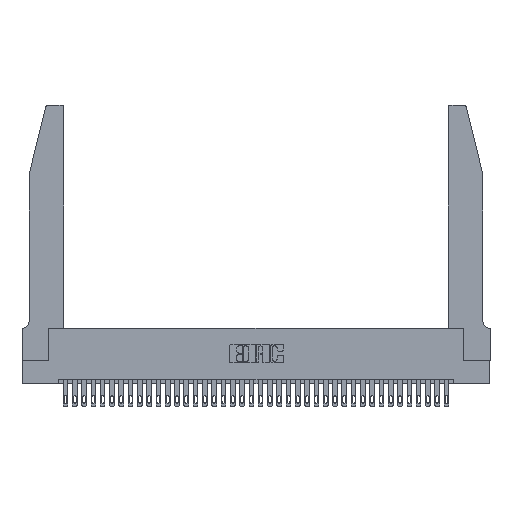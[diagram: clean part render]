
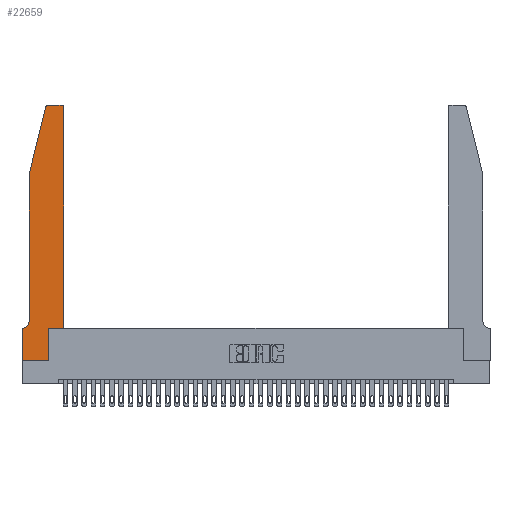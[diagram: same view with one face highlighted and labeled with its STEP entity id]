
A CAD part, top view. The second image highlights one B-rep face of the part: STEP entity #22659.
In plain terms, the highlighted planar face has unit normal (0, 0, 1).
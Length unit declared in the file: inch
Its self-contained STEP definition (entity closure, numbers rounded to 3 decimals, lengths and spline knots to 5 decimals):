
#34 = CARTESIAN_POINT ( 'NONE',  ( 0.2865, 0.35, 0.37 ) ) ;
#37 = VECTOR ( 'NONE', #2046, 39.37008 ) ;
#203 = DIRECTION ( 'NONE',  ( 0., -1., 0. ) ) ;
#481 = DIRECTION ( 'NONE',  ( 1., 0., 0. ) ) ;
#1280 = DIRECTION ( 'NONE',  ( 1., 0., 0. ) ) ;
#1301 = EDGE_LOOP ( 'NONE', ( #9736, #4219, #26477, #19954, #29222, #14273, #37280, #23417, #18162, #31074, #12852, #13388 ) ) ;
#1798 = DIRECTION ( 'NONE',  ( 0., 0., 1. ) ) ;
#1850 = CARTESIAN_POINT ( 'NONE',  ( 0.2865, 0.35, 0.37 ) ) ;
#2046 = DIRECTION ( 'NONE',  ( -1., 0., 0. ) ) ;
#2062 = DIRECTION ( 'NONE',  ( 0., -1., 0. ) ) ;
#2113 = VERTEX_POINT ( 'NONE', #24367 ) ;
#2620 = EDGE_CURVE ( 'NONE', #37609, #18117, #11911, .T. ) ;
#4219 = ORIENTED_EDGE ( 'NONE', *, *, #23172, .T. ) ;
#4554 = CARTESIAN_POINT ( 'NONE',  ( 0.0755, 0.35, 0.37 ) ) ;
#5546 = CARTESIAN_POINT ( 'NONE',  ( 0.0755, 2., 0.37 ) ) ;
#5962 = EDGE_CURVE ( 'NONE', #24337, #14425, #37158, .T. ) ;
#6208 = VERTEX_POINT ( 'NONE', #29455 ) ;
#6358 = EDGE_CURVE ( 'NONE', #33517, #25069, #22091, .T. ) ;
#6858 = FACE_OUTER_BOUND ( 'NONE', #1301, .T. ) ;
#7164 = CARTESIAN_POINT ( 'NONE',  ( 0.0055, 0.35, 0.37 ) ) ;
#7223 = EDGE_CURVE ( 'NONE', #18117, #29680, #34814, .T. ) ;
#7551 = VECTOR ( 'NONE', #13988, 39.37008 ) ;
#7570 = DIRECTION ( 'NONE',  ( 0., 1., 0. ) ) ;
#8617 = LINE ( 'NONE', #17896, #35463 ) ;
#8846 = VERTEX_POINT ( 'NONE', #34 ) ;
#9012 = VECTOR ( 'NONE', #7570, 39.37008 ) ;
#9397 = CARTESIAN_POINT ( 'NONE',  ( 0., 0.35, 0.37 ) ) ;
#9736 = ORIENTED_EDGE ( 'NONE', *, *, #22976, .T. ) ;
#9951 = EDGE_CURVE ( 'NONE', #8846, #37609, #8617, .T. ) ;
#10665 = DIRECTION ( 'NONE',  ( 1., 0., 0. ) ) ;
#10970 = CARTESIAN_POINT ( 'NONE',  ( 0.2865, 0., 0.37 ) ) ;
#11334 = AXIS2_PLACEMENT_3D ( 'NONE', #11372, #22546, #16957 ) ;
#11372 = CARTESIAN_POINT ( 'NONE',  ( 0.0055, 0.42, 0.37 ) ) ;
#11835 = AXIS2_PLACEMENT_3D ( 'NONE', #34987, #29153, #35109 ) ;
#11911 = LINE ( 'NONE', #20612, #34189 ) ;
#12852 = ORIENTED_EDGE ( 'NONE', *, *, #2620, .T. ) ;
#13388 = ORIENTED_EDGE ( 'NONE', *, *, #7223, .T. ) ;
#13587 = EDGE_CURVE ( 'NONE', #14425, #22671, #31050, .T. ) ;
#13988 = DIRECTION ( 'NONE',  ( 1., 0., 0. ) ) ;
#14273 = ORIENTED_EDGE ( 'NONE', *, *, #13587, .T. ) ;
#14425 = VERTEX_POINT ( 'NONE', #7164 ) ;
#14853 = LINE ( 'NONE', #17844, #16648 ) ;
#15024 = PLANE ( 'NONE',  #11835 ) ;
#15440 = CARTESIAN_POINT ( 'NONE',  ( 0.4505, 0.35, 0.37 ) ) ;
#15994 = EDGE_CURVE ( 'NONE', #6208, #23126, #14853, .T. ) ;
#16648 = VECTOR ( 'NONE', #33092, 39.37008 ) ;
#16957 = DIRECTION ( 'NONE',  ( -1., 0., 0. ) ) ;
#17554 = CARTESIAN_POINT ( 'NONE',  ( 0., 0., 0.37 ) ) ;
#17844 = CARTESIAN_POINT ( 'NONE',  ( 0.0755, 2., 0.37 ) ) ;
#17896 = CARTESIAN_POINT ( 'NONE',  ( 0.4505, 0.35, 0.37 ) ) ;
#18117 = VERTEX_POINT ( 'NONE', #36304 ) ;
#18162 = ORIENTED_EDGE ( 'NONE', *, *, #24918, .T. ) ;
#18440 = CARTESIAN_POINT ( 'NONE',  ( 0.2605, 2.75, 0.37 ) ) ;
#18867 = AXIS2_PLACEMENT_3D ( 'NONE', #36766, #1798, #10665 ) ;
#19746 = EDGE_CURVE ( 'NONE', #23126, #24337, #34637, .T. ) ;
#19954 = ORIENTED_EDGE ( 'NONE', *, *, #19746, .T. ) ;
#20612 = CARTESIAN_POINT ( 'NONE',  ( 0.4505, 0.35, 0.37 ) ) ;
#22091 = LINE ( 'NONE', #34870, #7551 ) ;
#22546 = DIRECTION ( 'NONE',  ( 0., 0., -1. ) ) ;
#22659 = ADVANCED_FACE ( 'NONE', ( #6858 ), #15024, .T. ) ;
#22671 = VERTEX_POINT ( 'NONE', #9397 ) ;
#22976 = EDGE_CURVE ( 'NONE', #29680, #2113, #28690, .T. ) ;
#23126 = VERTEX_POINT ( 'NONE', #5546 ) ;
#23172 = EDGE_CURVE ( 'NONE', #2113, #6208, #29584, .T. ) ;
#23417 = ORIENTED_EDGE ( 'NONE', *, *, #6358, .T. ) ;
#24337 = VERTEX_POINT ( 'NONE', #27074 ) ;
#24367 = CARTESIAN_POINT ( 'NONE',  ( 0.284, 2.75, 0.37 ) ) ;
#24489 = DIRECTION ( 'NONE',  ( -1., 0., 0. ) ) ;
#24918 = EDGE_CURVE ( 'NONE', #25069, #8846, #29060, .T. ) ;
#25069 = VERTEX_POINT ( 'NONE', #10970 ) ;
#25308 = CARTESIAN_POINT ( 'NONE',  ( 0.0755, 2., 0.37 ) ) ;
#26477 = ORIENTED_EDGE ( 'NONE', *, *, #15994, .T. ) ;
#26687 = DIRECTION ( 'NONE',  ( 0., 1., 0. ) ) ;
#27074 = CARTESIAN_POINT ( 'NONE',  ( 0.0755, 0.42, 0.37 ) ) ;
#27546 = AXIS2_PLACEMENT_3D ( 'NONE', #33434, #36373, #1280 ) ;
#27767 = VECTOR ( 'NONE', #2062, 39.37008 ) ;
#27846 = EDGE_CURVE ( 'NONE', #22671, #33517, #32639, .T. ) ;
#27896 = CARTESIAN_POINT ( 'NONE',  ( 0., 0., 0.37 ) ) ;
#28690 = LINE ( 'NONE', #18440, #37 ) ;
#29060 = LINE ( 'NONE', #1850, #9012 ) ;
#29153 = DIRECTION ( 'NONE',  ( 0., 0., 1. ) ) ;
#29222 = ORIENTED_EDGE ( 'NONE', *, *, #5962, .T. ) ;
#29455 = CARTESIAN_POINT ( 'NONE',  ( 0.25487, 2.72718, 0.37 ) ) ;
#29584 = CIRCLE ( 'NONE', #18867, 0.03 ) ;
#29680 = VERTEX_POINT ( 'NONE', #30494 ) ;
#30494 = CARTESIAN_POINT ( 'NONE',  ( 0.4205, 2.75, 0.37 ) ) ;
#31050 = LINE ( 'NONE', #4554, #33322 ) ;
#31074 = ORIENTED_EDGE ( 'NONE', *, *, #9951, .T. ) ;
#31692 = VECTOR ( 'NONE', #203, 39.37008 ) ;
#32639 = LINE ( 'NONE', #27896, #31692 ) ;
#33092 = DIRECTION ( 'NONE',  ( -0.239, -0.971, 0. ) ) ;
#33322 = VECTOR ( 'NONE', #24489, 39.37008 ) ;
#33434 = CARTESIAN_POINT ( 'NONE',  ( 0.4205, 2.72, 0.37 ) ) ;
#33517 = VERTEX_POINT ( 'NONE', #17554 ) ;
#34189 = VECTOR ( 'NONE', #26687, 39.37008 ) ;
#34637 = LINE ( 'NONE', #25308, #27767 ) ;
#34814 = CIRCLE ( 'NONE', #27546, 0.03 ) ;
#34870 = CARTESIAN_POINT ( 'NONE',  ( 0., 0., 0.37 ) ) ;
#34987 = CARTESIAN_POINT ( 'NONE',  ( 0., 0.35, 0.37 ) ) ;
#35109 = DIRECTION ( 'NONE',  ( 1., 0., 0. ) ) ;
#35463 = VECTOR ( 'NONE', #481, 39.37008 ) ;
#36304 = CARTESIAN_POINT ( 'NONE',  ( 0.4505, 2.72, 0.37 ) ) ;
#36373 = DIRECTION ( 'NONE',  ( 0., 0., 1. ) ) ;
#36766 = CARTESIAN_POINT ( 'NONE',  ( 0.284, 2.72, 0.37 ) ) ;
#37158 = CIRCLE ( 'NONE', #11334, 0.07 ) ;
#37280 = ORIENTED_EDGE ( 'NONE', *, *, #27846, .T. ) ;
#37609 = VERTEX_POINT ( 'NONE', #15440 ) ;
